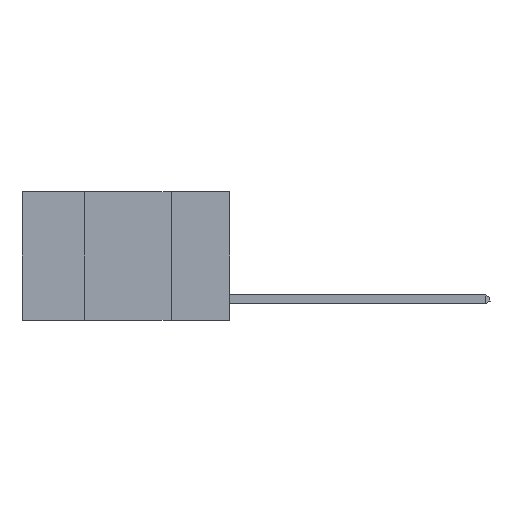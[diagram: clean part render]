
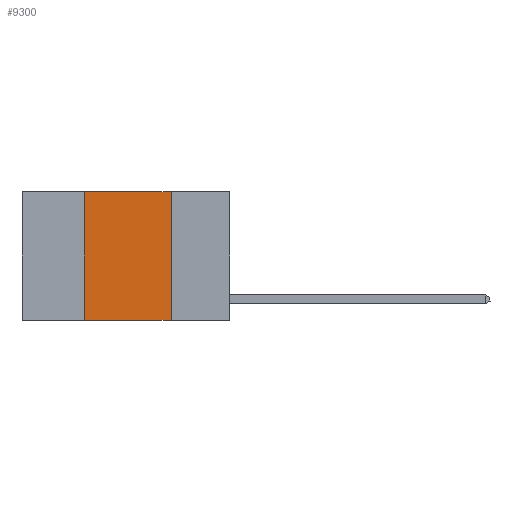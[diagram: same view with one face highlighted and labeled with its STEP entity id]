
A CAD part, left-side view. The second image highlights one B-rep face of the part: STEP entity #9300.
In plain terms, the highlighted planar face has unit normal (-1, 0, 0).
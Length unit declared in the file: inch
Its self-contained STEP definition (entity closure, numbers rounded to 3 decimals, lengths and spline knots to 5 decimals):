
#239 = DIRECTION ( 'NONE',  ( 0., -1., 0. ) ) ;
#536 = CARTESIAN_POINT ( 'NONE',  ( 0., 0.42, 0. ) ) ;
#578 = CARTESIAN_POINT ( 'NONE',  ( 0., 0.17, 0. ) ) ;
#933 = FACE_OUTER_BOUND ( 'NONE', #5820, .T. ) ;
#974 = AXIS2_PLACEMENT_3D ( 'NONE', #5640, #6784, #7619 ) ;
#1092 = CARTESIAN_POINT ( 'NONE',  ( 0., 0.6, -0.37 ) ) ;
#1508 = CARTESIAN_POINT ( 'NONE',  ( 0., 0.17, 0. ) ) ;
#1702 = PLANE ( 'NONE',  #974 ) ;
#1772 = VECTOR ( 'NONE', #239, 39.37008 ) ;
#2672 = VERTEX_POINT ( 'NONE', #578 ) ;
#2746 = DIRECTION ( 'NONE',  ( 0., -1., 0. ) ) ;
#2789 = CARTESIAN_POINT ( 'NONE',  ( 0., 0.42, 0. ) ) ;
#2861 = LINE ( 'NONE', #1092, #5261 ) ;
#3101 = CARTESIAN_POINT ( 'NONE',  ( 0., 0.17, -0.37 ) ) ;
#3237 = EDGE_CURVE ( 'NONE', #8628, #2672, #8531, .T. ) ;
#3917 = VECTOR ( 'NONE', #6429, 39.37008 ) ;
#4783 = DIRECTION ( 'NONE',  ( 0., 0., 1. ) ) ;
#5250 = ORIENTED_EDGE ( 'NONE', *, *, #5542, .F. ) ;
#5261 = VECTOR ( 'NONE', #2746, 39.37008 ) ;
#5542 = EDGE_CURVE ( 'NONE', #7465, #8628, #7167, .T. ) ;
#5640 = CARTESIAN_POINT ( 'NONE',  ( 0., 0.6, 0. ) ) ;
#5820 = EDGE_LOOP ( 'NONE', ( #9250, #9208, #5250, #6685 ) ) ;
#6429 = DIRECTION ( 'NONE',  ( 0., 0., -1. ) ) ;
#6481 = LINE ( 'NONE', #1508, #3917 ) ;
#6685 = ORIENTED_EDGE ( 'NONE', *, *, #8127, .T. ) ;
#6784 = DIRECTION ( 'NONE',  ( 1., 0., 0. ) ) ;
#6913 = CARTESIAN_POINT ( 'NONE',  ( 0., 0.6, 0. ) ) ;
#7167 = LINE ( 'NONE', #536, #9643 ) ;
#7404 = VERTEX_POINT ( 'NONE', #3101 ) ;
#7465 = VERTEX_POINT ( 'NONE', #8292 ) ;
#7619 = DIRECTION ( 'NONE',  ( 0., 0., -1. ) ) ;
#8127 = EDGE_CURVE ( 'NONE', #7465, #7404, #2861, .T. ) ;
#8292 = CARTESIAN_POINT ( 'NONE',  ( 0., 0.42, -0.37 ) ) ;
#8531 = LINE ( 'NONE', #6913, #1772 ) ;
#8628 = VERTEX_POINT ( 'NONE', #2789 ) ;
#8787 = EDGE_CURVE ( 'NONE', #2672, #7404, #6481, .T. ) ;
#9208 = ORIENTED_EDGE ( 'NONE', *, *, #3237, .F. ) ;
#9250 = ORIENTED_EDGE ( 'NONE', *, *, #8787, .F. ) ;
#9300 = ADVANCED_FACE ( 'NONE', ( #933 ), #1702, .F. ) ;
#9643 = VECTOR ( 'NONE', #4783, 39.37008 ) ;
